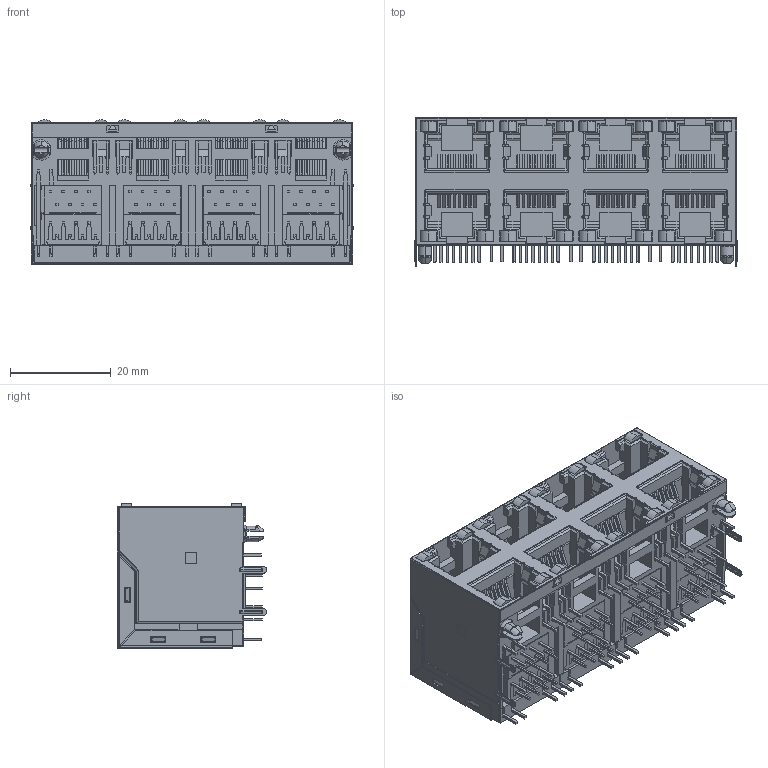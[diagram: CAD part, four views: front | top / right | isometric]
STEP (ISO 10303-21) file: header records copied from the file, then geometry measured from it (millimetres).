
FILE_DESCRIPTION (( 'STEP AP203' ), '1' );
FILE_NAME ('J96088892N41121.STEP', '2020-03-24T05:42:46', ( '' ), ( '' ), 'SwSTEP 2.0', 'SolidWorks 2016', '' );
FILE_SCHEMA (( 'CONFIG_CONTROL_DESIGN' ));
Length unit declared in the file: millimetre
Products named in the file (14): 96 LED RH Lower_1-Yellow; 96 Contacts Lower; 96 Insulator_8 Ports; 96 Back Plate_8 Ports; 96 Shield_8 Ports LED - No EMI; 96 Contact Lock Lower; 96 Contacts Upper; J96088892N41121; 96 LED LH Upper_4-Orange; 96 LED LH Lower_4-Orange; 96 Grounding_8 Ports; 96 Contact Lock Upper; 96 LED RH Upper_1-Yellow; 96 Insulator Insert
Assembly tree (40 placements, depth 2):
  J96088892N41121
    96 Insulator_8 Ports
    96 LED LH Lower_4-Orange  x4
    96 LED RH Lower_1-Yellow  x4
    96 Contacts Lower  x4
    96 Contact Lock Lower  x4
    96 Grounding_8 Ports
    96 Contacts Upper  x4
    96 Contact Lock Upper  x4
    96 Insulator Insert  x4
    96 LED LH Upper_4-Orange  x4
    96 LED RH Upper_1-Yellow  x4
    96 Back Plate_8 Ports
    96 Shield_8 Ports LED - No EMI
Bounding box: 64.05 x 29.58 x 28.68 mm (x, y, z)
Volume: 24160 mm3; surface area: 63657.9 mm2
Topology: 96 solids, 96 shells, 7642 faces, 21478 edges, 13802 vertices
Faces by surface type: plane 6069, cylinder 1307, bspline 252, cone 14
Entity records: 143018 total; most frequent: CARTESIAN_POINT 31500, ORIENTED_EDGE 24348, DIRECTION 20463, EDGE_CURVE 12174, VECTOR 9967, LINE 9967, VERTEX_POINT 7869, AXIS2_PLACEMENT_3D 5248
